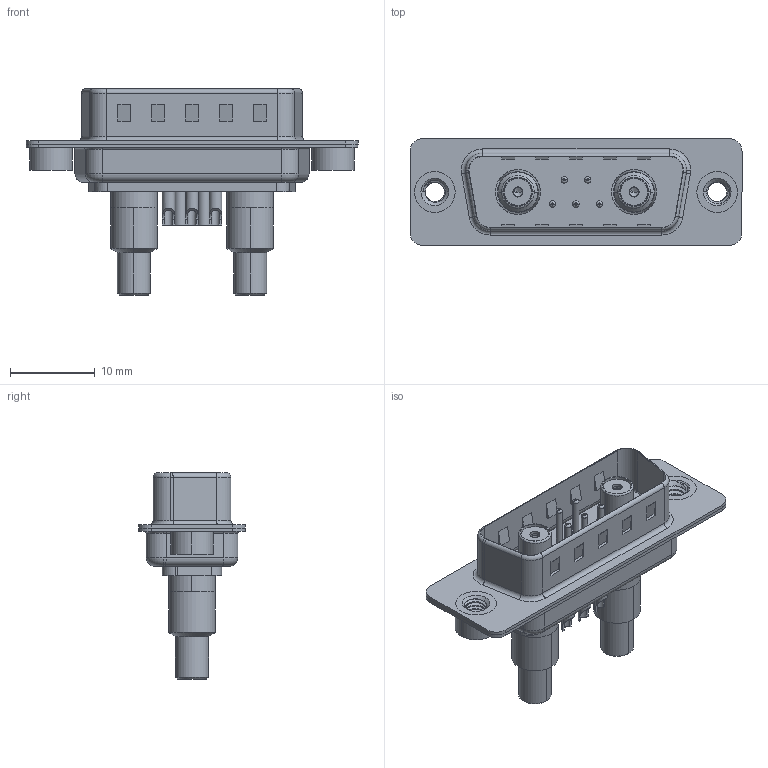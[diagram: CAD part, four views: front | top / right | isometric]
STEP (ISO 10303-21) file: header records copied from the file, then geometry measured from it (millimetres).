
FILE_DESCRIPTION (( 'STEP AP203' ), '1' );
FILE_NAME ('627-7W2-222-7TA.STEP', '2019-05-25T03:07:01', ( '' ), ( '' ), 'SwSTEP 2.0', 'SolidWorks 2016', '' );
FILE_SCHEMA (( 'CONFIG_CONTROL_DESIGN' ));
Length unit declared in the file: millimetre
Products named in the file (15): 627Combo Contact Row 2_22; Insulator Socket; 627-7W2-222-7TA; Insulator Socket 2; Locking Collar; Socket_Solder Cup; 627Combo Housing_7W2; Solder Cover; 627Combo Shell Rear_15 Contacts; Co-Ax Jack Assy_SC; 627Combo Shell Front_15 Contacts; 627Combo Threaded Rivet_2; 627Combo Threaded Rivet_A; 627Combo Contact Row 1_22; Co-Ax Jack_Solder Cup Tail
Assembly tree (18 placements, depth 3):
  627-7W2-222-7TA
    627Combo Housing_7W2
    627Combo Shell Rear_15 Contacts
    627Combo Shell Front_15 Contacts
    627Combo Threaded Rivet_A
    Co-Ax Jack Assy_SC  x2
      Co-Ax Jack_Solder Cup Tail
      Insulator Socket
      Insulator Socket 2
      Locking Collar
      Socket_Solder Cup
      Solder Cover
    627Combo Threaded Rivet_2
    627Combo Contact Row 1_22  x2
    627Combo Contact Row 2_22  x3
Bounding box: 39.15 x 12.6 x 24.3 mm (x, y, z)
Volume: 2105.9 mm3; surface area: 6456.3 mm2
Topology: 22 solids, 22 shells, 784 faces, 1852 edges, 1143 vertices
Faces by surface type: cylinder 342, plane 264, torus 108, cone 60, bspline 10
Entity records: 21686 total; most frequent: CARTESIAN_POINT 6361, DIRECTION 3019, ORIENTED_EDGE 2734, EDGE_CURVE 1367, AXIS2_PLACEMENT_3D 1179, VERTEX_POINT 858, EDGE_LOOP 669, VECTOR 661
